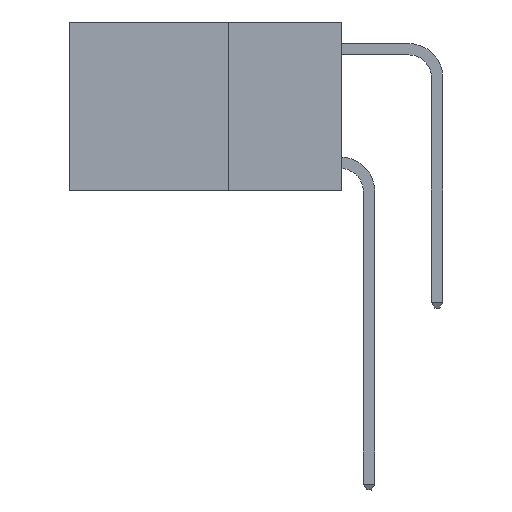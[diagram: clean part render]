
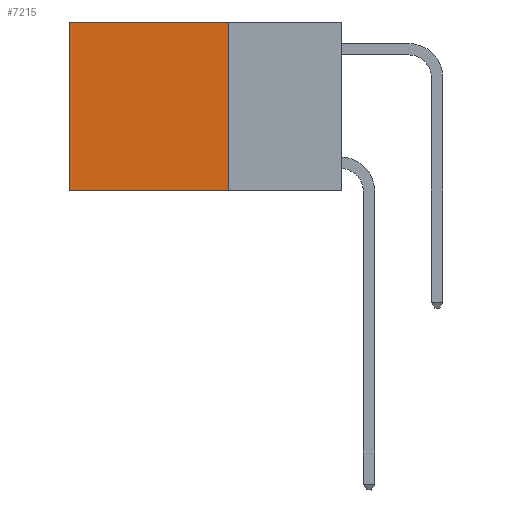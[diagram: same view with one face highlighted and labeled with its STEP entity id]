
A CAD part, left-side view. The second image highlights one B-rep face of the part: STEP entity #7215.
In plain terms, the highlighted planar face has unit normal (-1, 0, 0).
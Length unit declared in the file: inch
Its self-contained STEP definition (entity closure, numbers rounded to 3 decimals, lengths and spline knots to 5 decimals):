
#503 = FACE_OUTER_BOUND ( 'NONE', #1074, .T. ) ;
#655 = EDGE_CURVE ( 'NONE', #6324, #4780, #8458, .T. ) ;
#1074 = EDGE_LOOP ( 'NONE', ( #8630, #2872, #10959, #3042 ) ) ;
#1531 = EDGE_CURVE ( 'NONE', #4780, #11144, #2673, .T. ) ;
#1564 = LINE ( 'NONE', #8814, #8624 ) ;
#1853 = CARTESIAN_POINT ( 'NONE',  ( 0.2625, 0.25, 0. ) ) ;
#2222 = LINE ( 'NONE', #3949, #4517 ) ;
#2673 = LINE ( 'NONE', #11295, #5236 ) ;
#2872 = ORIENTED_EDGE ( 'NONE', *, *, #11601, .F. ) ;
#3042 = ORIENTED_EDGE ( 'NONE', *, *, #655, .T. ) ;
#3949 = CARTESIAN_POINT ( 'NONE',  ( 0.2625, 0.25, -0.37 ) ) ;
#4336 = CARTESIAN_POINT ( 'NONE',  ( 0.2625, 0.25, 0. ) ) ;
#4517 = VECTOR ( 'NONE', #4878, 39.37008 ) ;
#4780 = VERTEX_POINT ( 'NONE', #5745 ) ;
#4878 = DIRECTION ( 'NONE',  ( 0., 1., 0. ) ) ;
#5230 = CARTESIAN_POINT ( 'NONE',  ( 0.2625, 0.6, -0.37 ) ) ;
#5236 = VECTOR ( 'NONE', #12124, 39.37008 ) ;
#5307 = DIRECTION ( 'NONE',  ( 0., 0., -1. ) ) ;
#5586 = CARTESIAN_POINT ( 'NONE',  ( 0.2625, 0.25, -0.37 ) ) ;
#5745 = CARTESIAN_POINT ( 'NONE',  ( 0.2625, 0.6, 0. ) ) ;
#6324 = VERTEX_POINT ( 'NONE', #1853 ) ;
#6595 = EDGE_CURVE ( 'NONE', #6324, #11435, #1564, .T. ) ;
#7044 = DIRECTION ( 'NONE',  ( 0., 0., -1. ) ) ;
#7215 = ADVANCED_FACE ( 'NONE', ( #503 ), #9904, .F. ) ;
#7526 = DIRECTION ( 'NONE',  ( 0., 1., 0. ) ) ;
#7539 = CARTESIAN_POINT ( 'NONE',  ( 0.2625, 0.25, 0. ) ) ;
#8458 = LINE ( 'NONE', #7539, #10003 ) ;
#8624 = VECTOR ( 'NONE', #7044, 39.37008 ) ;
#8630 = ORIENTED_EDGE ( 'NONE', *, *, #1531, .T. ) ;
#8814 = CARTESIAN_POINT ( 'NONE',  ( 0.2625, 0.25, 0. ) ) ;
#9904 = PLANE ( 'NONE',  #10028 ) ;
#10003 = VECTOR ( 'NONE', #7526, 39.37008 ) ;
#10028 = AXIS2_PLACEMENT_3D ( 'NONE', #4336, #10752, #5307 ) ;
#10752 = DIRECTION ( 'NONE',  ( 1., 0., 0. ) ) ;
#10959 = ORIENTED_EDGE ( 'NONE', *, *, #6595, .F. ) ;
#11144 = VERTEX_POINT ( 'NONE', #5230 ) ;
#11295 = CARTESIAN_POINT ( 'NONE',  ( 0.2625, 0.6, 0. ) ) ;
#11435 = VERTEX_POINT ( 'NONE', #5586 ) ;
#11601 = EDGE_CURVE ( 'NONE', #11435, #11144, #2222, .T. ) ;
#12124 = DIRECTION ( 'NONE',  ( 0., 0., -1. ) ) ;
